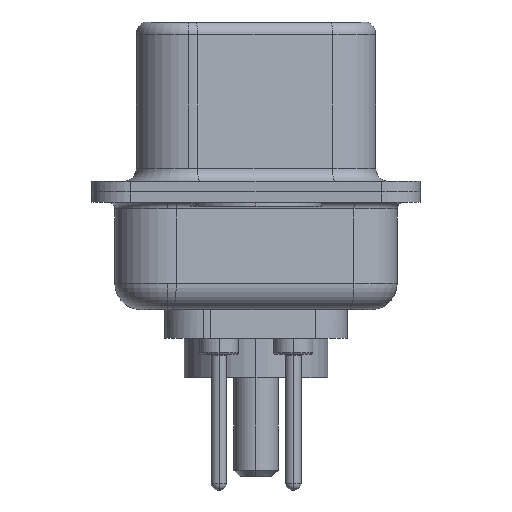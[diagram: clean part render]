
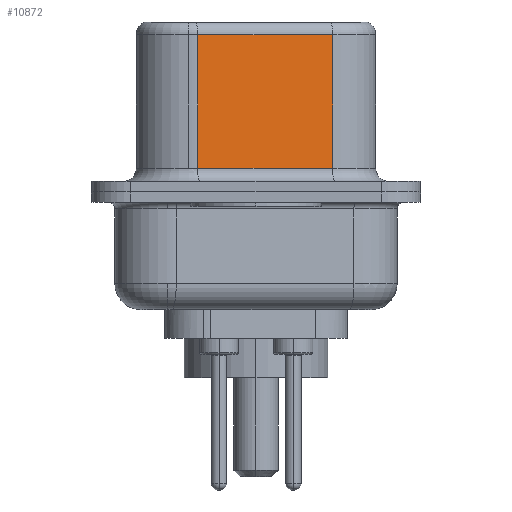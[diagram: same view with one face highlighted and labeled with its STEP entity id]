
A CAD part, left-side view. The second image highlights one B-rep face of the part: STEP entity #10872.
In plain terms, the highlighted planar face has unit normal (-0.985, -0.174, 0).
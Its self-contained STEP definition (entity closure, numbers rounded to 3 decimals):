
#68 = ORIENTED_EDGE ( 'NONE', *, *, #1614, .T. ) ;
#104 = DIRECTION ( 'NONE',  ( -0.174, 0.985, 0. ) ) ;
#221 = VERTEX_POINT ( 'NONE', #9988 ) ;
#822 = LINE ( 'NONE', #5291, #3065 ) ;
#1113 = VECTOR ( 'NONE', #11792, 1000. ) ;
#1614 = EDGE_CURVE ( 'NONE', #5063, #5539, #3686, .T. ) ;
#1654 = EDGE_CURVE ( 'NONE', #8264, #5539, #822, .T. ) ;
#2248 = VECTOR ( 'NONE', #7019, 1000. ) ;
#2410 = DIRECTION ( 'NONE',  ( -0.174, 0.985, 0. ) ) ;
#2437 = LINE ( 'NONE', #4908, #4361 ) ;
#3065 = VECTOR ( 'NONE', #4314, 1000. ) ;
#3346 = ORIENTED_EDGE ( 'NONE', *, *, #3647, .T. ) ;
#3647 = EDGE_CURVE ( 'NONE', #8264, #221, #2437, .T. ) ;
#3686 = LINE ( 'NONE', #9484, #1113 ) ;
#4314 = DIRECTION ( 'NONE',  ( 0., 0., -1. ) ) ;
#4361 = VECTOR ( 'NONE', #104, 1000. ) ;
#4663 = CARTESIAN_POINT ( 'NONE',  ( 4.58, -2.927, 6.02 ) ) ;
#4770 = CARTESIAN_POINT ( 'NONE',  ( 3.67, 2.233, 6.52 ) ) ;
#4908 = CARTESIAN_POINT ( 'NONE',  ( 4.58, -2.927, 6.02 ) ) ;
#5063 = VERTEX_POINT ( 'NONE', #8998 ) ;
#5291 = CARTESIAN_POINT ( 'NONE',  ( 4.58, -2.927, 6.52 ) ) ;
#5436 = EDGE_CURVE ( 'NONE', #221, #5063, #11899, .T. ) ;
#5539 = VERTEX_POINT ( 'NONE', #9675 ) ;
#5898 = ORIENTED_EDGE ( 'NONE', *, *, #5436, .T. ) ;
#6139 = CARTESIAN_POINT ( 'NONE',  ( 4.58, -2.927, 6.52 ) ) ;
#7019 = DIRECTION ( 'NONE',  ( 0., 0., -1. ) ) ;
#8009 = DIRECTION ( 'NONE',  ( 0.985, 0.174, 0. ) ) ;
#8264 = VERTEX_POINT ( 'NONE', #4663 ) ;
#8998 = CARTESIAN_POINT ( 'NONE',  ( 3.67, 2.233, 0.9 ) ) ;
#9450 = AXIS2_PLACEMENT_3D ( 'NONE', #6139, #8009, #2410 ) ;
#9484 = CARTESIAN_POINT ( 'NONE',  ( 4.58, -2.927, 0.9 ) ) ;
#9675 = CARTESIAN_POINT ( 'NONE',  ( 4.58, -2.927, 0.9 ) ) ;
#9853 = PLANE ( 'NONE',  #9450 ) ;
#9896 = ORIENTED_EDGE ( 'NONE', *, *, #1654, .F. ) ;
#9988 = CARTESIAN_POINT ( 'NONE',  ( 3.67, 2.233, 6.02 ) ) ;
#10163 = EDGE_LOOP ( 'NONE', ( #9896, #3346, #5898, #68 ) ) ;
#10872 = ADVANCED_FACE ( 'NONE', ( #11911 ), #9853, .F. ) ;
#11792 = DIRECTION ( 'NONE',  ( 0.174, -0.985, 0. ) ) ;
#11899 = LINE ( 'NONE', #4770, #2248 ) ;
#11911 = FACE_OUTER_BOUND ( 'NONE', #10163, .T. ) ;
